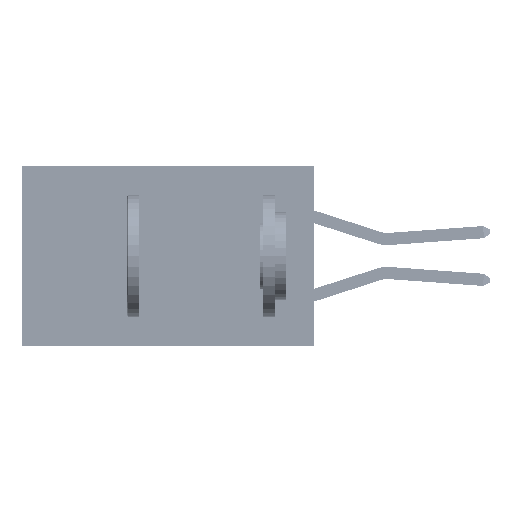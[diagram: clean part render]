
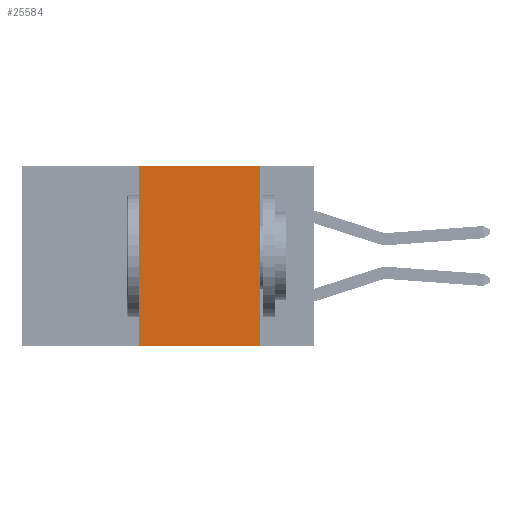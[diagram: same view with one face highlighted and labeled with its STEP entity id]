
A CAD part, left-side view. The second image highlights one B-rep face of the part: STEP entity #25584.
In plain terms, the highlighted planar face has unit normal (-1, 0, 0).
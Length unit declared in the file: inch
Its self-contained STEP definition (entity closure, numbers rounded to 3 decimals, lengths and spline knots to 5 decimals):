
#2520 = DIRECTION ( 'NONE',  ( 0., -1., 0. ) ) ;
#3600 = CARTESIAN_POINT ( 'NONE',  ( 0., 0.36, 0. ) ) ;
#6504 = CARTESIAN_POINT ( 'NONE',  ( 0., 0.11, -0.37 ) ) ;
#6791 = DIRECTION ( 'NONE',  ( 1., 0., 0. ) ) ;
#7459 = ORIENTED_EDGE ( 'NONE', *, *, #13719, .F. ) ;
#7512 = VERTEX_POINT ( 'NONE', #3600 ) ;
#7919 = VECTOR ( 'NONE', #2520, 39.37008 ) ;
#9054 = DIRECTION ( 'NONE',  ( 0., 0., -1. ) ) ;
#10928 = VECTOR ( 'NONE', #47124, 39.37008 ) ;
#11423 = LINE ( 'NONE', #21458, #35576 ) ;
#11938 = VERTEX_POINT ( 'NONE', #6504 ) ;
#13719 = EDGE_CURVE ( 'NONE', #44170, #11938, #29412, .T. ) ;
#15391 = EDGE_LOOP ( 'NONE', ( #7459, #17835, #18256, #21278 ) ) ;
#17383 = CARTESIAN_POINT ( 'NONE',  ( 0., 0.6, 0. ) ) ;
#17835 = ORIENTED_EDGE ( 'NONE', *, *, #45882, .F. ) ;
#18256 = ORIENTED_EDGE ( 'NONE', *, *, #27487, .F. ) ;
#19511 = EDGE_CURVE ( 'NONE', #33812, #11938, #37212, .T. ) ;
#19690 = CARTESIAN_POINT ( 'NONE',  ( 0., 0.11, 0. ) ) ;
#21278 = ORIENTED_EDGE ( 'NONE', *, *, #19511, .T. ) ;
#21458 = CARTESIAN_POINT ( 'NONE',  ( 0., 0.36, 0. ) ) ;
#21515 = CARTESIAN_POINT ( 'NONE',  ( 0., 0.6, 0. ) ) ;
#25584 = ADVANCED_FACE ( 'NONE', ( #27708 ), #43685, .F. ) ;
#27487 = EDGE_CURVE ( 'NONE', #33812, #7512, #11423, .T. ) ;
#27708 = FACE_OUTER_BOUND ( 'NONE', #15391, .T. ) ;
#29412 = LINE ( 'NONE', #19690, #36875 ) ;
#31750 = CARTESIAN_POINT ( 'NONE',  ( 0., 0.6, -0.37 ) ) ;
#33812 = VERTEX_POINT ( 'NONE', #45240 ) ;
#35576 = VECTOR ( 'NONE', #40014, 39.37008 ) ;
#36875 = VECTOR ( 'NONE', #9054, 39.37008 ) ;
#37212 = LINE ( 'NONE', #31750, #7919 ) ;
#40014 = DIRECTION ( 'NONE',  ( 0., 0., 1. ) ) ;
#40197 = LINE ( 'NONE', #21515, #10928 ) ;
#43517 = CARTESIAN_POINT ( 'NONE',  ( 0., 0.11, 0. ) ) ;
#43685 = PLANE ( 'NONE',  #47254 ) ;
#44170 = VERTEX_POINT ( 'NONE', #43517 ) ;
#45240 = CARTESIAN_POINT ( 'NONE',  ( 0., 0.36, -0.37 ) ) ;
#45882 = EDGE_CURVE ( 'NONE', #7512, #44170, #40197, .T. ) ;
#46723 = DIRECTION ( 'NONE',  ( 0., 0., -1. ) ) ;
#47124 = DIRECTION ( 'NONE',  ( 0., -1., 0. ) ) ;
#47254 = AXIS2_PLACEMENT_3D ( 'NONE', #17383, #6791, #46723 ) ;
